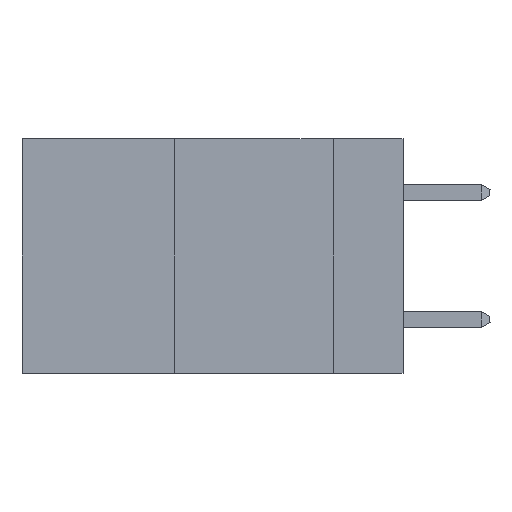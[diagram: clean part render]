
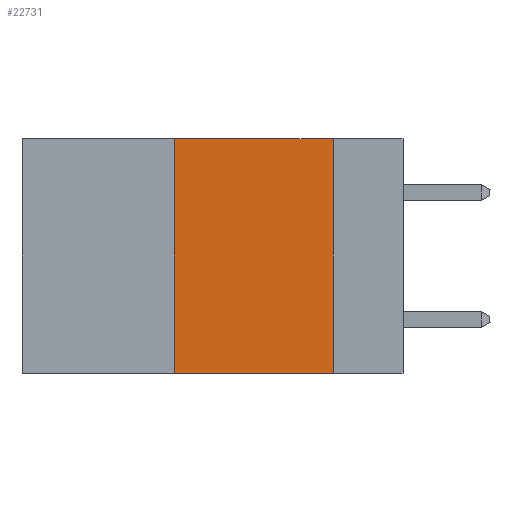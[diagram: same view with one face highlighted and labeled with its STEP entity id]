
A CAD part, left-side view. The second image highlights one B-rep face of the part: STEP entity #22731.
In plain terms, the highlighted planar face has unit normal (-1, 0, 0).
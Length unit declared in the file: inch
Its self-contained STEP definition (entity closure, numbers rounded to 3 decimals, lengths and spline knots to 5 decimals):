
#963 = VERTEX_POINT ( 'NONE', #7204 ) ;
#1138 = VERTEX_POINT ( 'NONE', #12701 ) ;
#1360 = VECTOR ( 'NONE', #22516, 39.37008 ) ;
#2322 = CARTESIAN_POINT ( 'NONE',  ( 0., 0.36, 0. ) ) ;
#3734 = CARTESIAN_POINT ( 'NONE',  ( 0., 0.36, 0. ) ) ;
#4200 = EDGE_CURVE ( 'NONE', #9318, #1138, #21400, .T. ) ;
#4453 = CARTESIAN_POINT ( 'NONE',  ( 0., 0.11, 0. ) ) ;
#4783 = EDGE_CURVE ( 'NONE', #23239, #9318, #12365, .T. ) ;
#5218 = LINE ( 'NONE', #17973, #29923 ) ;
#6959 = AXIS2_PLACEMENT_3D ( 'NONE', #28363, #14149, #30750 ) ;
#7182 = DIRECTION ( 'NONE',  ( 0., 0., 1. ) ) ;
#7204 = CARTESIAN_POINT ( 'NONE',  ( 0., 0.36, -0.37 ) ) ;
#8091 = CARTESIAN_POINT ( 'NONE',  ( 0., 0.11, 0. ) ) ;
#9318 = VERTEX_POINT ( 'NONE', #4453 ) ;
#9407 = EDGE_CURVE ( 'NONE', #963, #23239, #24336, .T. ) ;
#12192 = EDGE_LOOP ( 'NONE', ( #30217, #26879, #21525, #15654 ) ) ;
#12365 = LINE ( 'NONE', #17286, #25075 ) ;
#12701 = CARTESIAN_POINT ( 'NONE',  ( 0., 0.11, -0.37 ) ) ;
#14149 = DIRECTION ( 'NONE',  ( 1., 0., 0. ) ) ;
#14856 = DIRECTION ( 'NONE',  ( 0., -1., 0. ) ) ;
#14901 = EDGE_CURVE ( 'NONE', #963, #1138, #5218, .T. ) ;
#15329 = FACE_OUTER_BOUND ( 'NONE', #12192, .T. ) ;
#15654 = ORIENTED_EDGE ( 'NONE', *, *, #14901, .T. ) ;
#17286 = CARTESIAN_POINT ( 'NONE',  ( 0., 0.6, 0. ) ) ;
#17973 = CARTESIAN_POINT ( 'NONE',  ( 0., 0.6, -0.37 ) ) ;
#18078 = VECTOR ( 'NONE', #7182, 39.37008 ) ;
#21285 = PLANE ( 'NONE',  #6959 ) ;
#21400 = LINE ( 'NONE', #8091, #1360 ) ;
#21525 = ORIENTED_EDGE ( 'NONE', *, *, #9407, .F. ) ;
#22516 = DIRECTION ( 'NONE',  ( 0., 0., -1. ) ) ;
#22731 = ADVANCED_FACE ( 'NONE', ( #15329 ), #21285, .F. ) ;
#23239 = VERTEX_POINT ( 'NONE', #3734 ) ;
#24336 = LINE ( 'NONE', #2322, #18078 ) ;
#25075 = VECTOR ( 'NONE', #14856, 39.37008 ) ;
#26879 = ORIENTED_EDGE ( 'NONE', *, *, #4783, .F. ) ;
#28363 = CARTESIAN_POINT ( 'NONE',  ( 0., 0.6, 0. ) ) ;
#29826 = DIRECTION ( 'NONE',  ( 0., -1., 0. ) ) ;
#29923 = VECTOR ( 'NONE', #29826, 39.37008 ) ;
#30217 = ORIENTED_EDGE ( 'NONE', *, *, #4200, .F. ) ;
#30750 = DIRECTION ( 'NONE',  ( 0., 0., -1. ) ) ;
